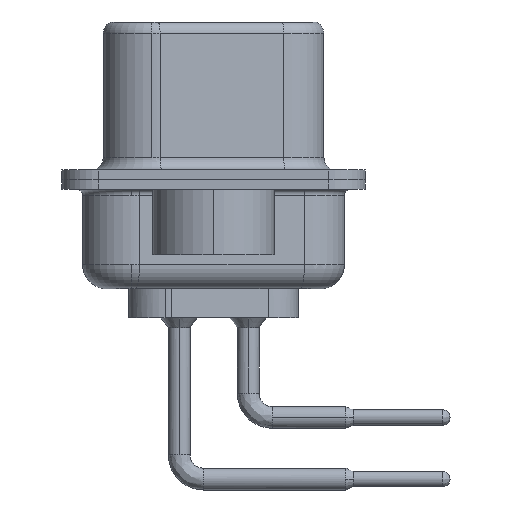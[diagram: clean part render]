
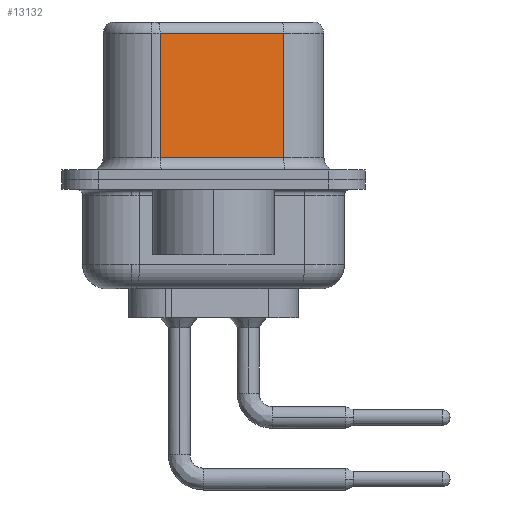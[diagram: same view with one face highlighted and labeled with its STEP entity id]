
A CAD part, left-side view. The second image highlights one B-rep face of the part: STEP entity #13132.
In plain terms, the highlighted planar face has unit normal (-0.985, -0.174, 0).
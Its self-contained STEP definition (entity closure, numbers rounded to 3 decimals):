
#585 = CARTESIAN_POINT ( 'NONE',  ( 4.58, -2.897, 6.52 ) ) ;
#600 = CARTESIAN_POINT ( 'NONE',  ( 4.58, -2.897, 0.9 ) ) ;
#2057 = CARTESIAN_POINT ( 'NONE',  ( 4.58, -2.897, 0.9 ) ) ;
#2149 = DIRECTION ( 'NONE',  ( 0.174, -0.985, 0. ) ) ;
#3752 = VECTOR ( 'NONE', #9584, 1000. ) ;
#3805 = CARTESIAN_POINT ( 'NONE',  ( 3.68, 2.203, 6.52 ) ) ;
#4326 = VERTEX_POINT ( 'NONE', #20536 ) ;
#4939 = EDGE_LOOP ( 'NONE', ( #20061, #12222, #23858, #14850 ) ) ;
#5212 = LINE ( 'NONE', #585, #15281 ) ;
#5863 = VECTOR ( 'NONE', #21602, 1000. ) ;
#6165 = EDGE_CURVE ( 'NONE', #4326, #21614, #9135, .T. ) ;
#6457 = CARTESIAN_POINT ( 'NONE',  ( 3.68, 2.203, 0.9 ) ) ;
#6940 = VECTOR ( 'NONE', #2149, 1000. ) ;
#8615 = FACE_OUTER_BOUND ( 'NONE', #4939, .T. ) ;
#9135 = LINE ( 'NONE', #13081, #3752 ) ;
#9317 = CARTESIAN_POINT ( 'NONE',  ( 4.58, -2.897, 6.52 ) ) ;
#9584 = DIRECTION ( 'NONE',  ( -0.174, 0.985, 0. ) ) ;
#11231 = LINE ( 'NONE', #3805, #5863 ) ;
#11391 = EDGE_CURVE ( 'NONE', #21614, #12259, #11231, .T. ) ;
#12222 = ORIENTED_EDGE ( 'NONE', *, *, #6165, .T. ) ;
#12259 = VERTEX_POINT ( 'NONE', #6457 ) ;
#13081 = CARTESIAN_POINT ( 'NONE',  ( 4.58, -2.897, 6.02 ) ) ;
#13132 = ADVANCED_FACE ( 'NONE', ( #8615 ), #22995, .F. ) ;
#13379 = DIRECTION ( 'NONE',  ( -0.174, 0.985, 0. ) ) ;
#14162 = CARTESIAN_POINT ( 'NONE',  ( 3.68, 2.203, 6.02 ) ) ;
#14515 = VERTEX_POINT ( 'NONE', #600 ) ;
#14850 = ORIENTED_EDGE ( 'NONE', *, *, #16153, .T. ) ;
#14916 = AXIS2_PLACEMENT_3D ( 'NONE', #9317, #25006, #13379 ) ;
#15281 = VECTOR ( 'NONE', #24570, 1000. ) ;
#16153 = EDGE_CURVE ( 'NONE', #12259, #14515, #21955, .T. ) ;
#20061 = ORIENTED_EDGE ( 'NONE', *, *, #20153, .F. ) ;
#20153 = EDGE_CURVE ( 'NONE', #4326, #14515, #5212, .T. ) ;
#20536 = CARTESIAN_POINT ( 'NONE',  ( 4.58, -2.897, 6.02 ) ) ;
#21602 = DIRECTION ( 'NONE',  ( 0., 0., -1. ) ) ;
#21614 = VERTEX_POINT ( 'NONE', #14162 ) ;
#21955 = LINE ( 'NONE', #2057, #6940 ) ;
#22995 = PLANE ( 'NONE',  #14916 ) ;
#23858 = ORIENTED_EDGE ( 'NONE', *, *, #11391, .T. ) ;
#24570 = DIRECTION ( 'NONE',  ( 0., 0., -1. ) ) ;
#25006 = DIRECTION ( 'NONE',  ( 0.985, 0.174, 0. ) ) ;
